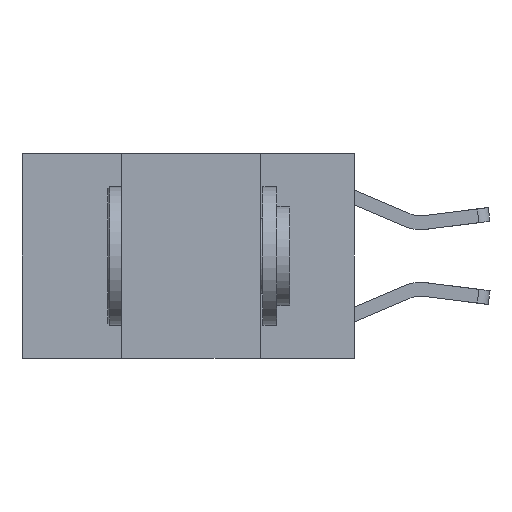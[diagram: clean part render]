
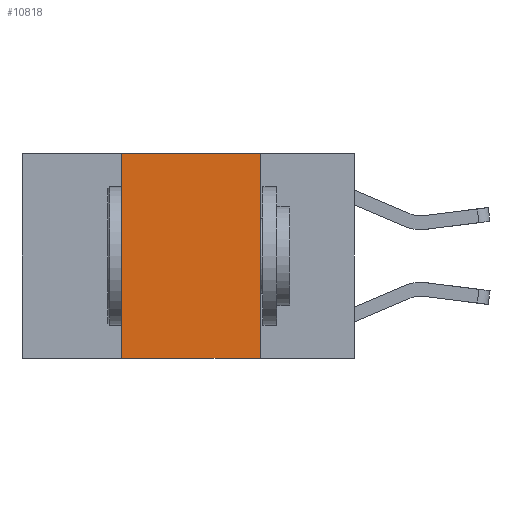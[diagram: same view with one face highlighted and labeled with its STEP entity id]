
A CAD part, left-side view. The second image highlights one B-rep face of the part: STEP entity #10818.
In plain terms, the highlighted planar face has unit normal (-1, 0, 0).
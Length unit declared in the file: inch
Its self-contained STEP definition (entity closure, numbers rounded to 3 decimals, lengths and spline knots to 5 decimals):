
#164 = PLANE ( 'NONE',  #9741 ) ;
#352 = LINE ( 'NONE', #2138, #2866 ) ;
#410 = ORIENTED_EDGE ( 'NONE', *, *, #660, .T. ) ;
#660 = EDGE_CURVE ( 'NONE', #4712, #5488, #6547, .T. ) ;
#1065 = EDGE_LOOP ( 'NONE', ( #1125, #4138, #1600, #410 ) ) ;
#1125 = ORIENTED_EDGE ( 'NONE', *, *, #5819, .F. ) ;
#1174 = DIRECTION ( 'NONE',  ( 0., 0., -1. ) ) ;
#1600 = ORIENTED_EDGE ( 'NONE', *, *, #7904, .F. ) ;
#2138 = CARTESIAN_POINT ( 'NONE',  ( 0., 0.6, 0. ) ) ;
#2260 = CARTESIAN_POINT ( 'NONE',  ( 0., 0.17, 0. ) ) ;
#2429 = DIRECTION ( 'NONE',  ( 0., -1., 0. ) ) ;
#2845 = EDGE_CURVE ( 'NONE', #5716, #3386, #352, .T. ) ;
#2866 = VECTOR ( 'NONE', #2429, 39.37008 ) ;
#3131 = DIRECTION ( 'NONE',  ( 0., 0., -1. ) ) ;
#3260 = CARTESIAN_POINT ( 'NONE',  ( 0., 0.17, 0. ) ) ;
#3386 = VERTEX_POINT ( 'NONE', #3260 ) ;
#3578 = DIRECTION ( 'NONE',  ( 0., 0., 1. ) ) ;
#4138 = ORIENTED_EDGE ( 'NONE', *, *, #2845, .F. ) ;
#4712 = VERTEX_POINT ( 'NONE', #9604 ) ;
#4734 = LINE ( 'NONE', #8833, #7087 ) ;
#5488 = VERTEX_POINT ( 'NONE', #9739 ) ;
#5716 = VERTEX_POINT ( 'NONE', #7437 ) ;
#5819 = EDGE_CURVE ( 'NONE', #3386, #5488, #9512, .T. ) ;
#6547 = LINE ( 'NONE', #10647, #8536 ) ;
#6597 = DIRECTION ( 'NONE',  ( 1., 0., 0. ) ) ;
#6972 = DIRECTION ( 'NONE',  ( 0., -1., 0. ) ) ;
#7087 = VECTOR ( 'NONE', #3578, 39.37008 ) ;
#7437 = CARTESIAN_POINT ( 'NONE',  ( 0., 0.42, 0. ) ) ;
#7904 = EDGE_CURVE ( 'NONE', #4712, #5716, #4734, .T. ) ;
#7917 = FACE_OUTER_BOUND ( 'NONE', #1065, .T. ) ;
#8536 = VECTOR ( 'NONE', #6972, 39.37008 ) ;
#8833 = CARTESIAN_POINT ( 'NONE',  ( 0., 0.42, 0. ) ) ;
#9512 = LINE ( 'NONE', #2260, #11208 ) ;
#9604 = CARTESIAN_POINT ( 'NONE',  ( 0., 0.42, -0.37 ) ) ;
#9739 = CARTESIAN_POINT ( 'NONE',  ( 0., 0.17, -0.37 ) ) ;
#9741 = AXIS2_PLACEMENT_3D ( 'NONE', #10815, #6597, #1174 ) ;
#10647 = CARTESIAN_POINT ( 'NONE',  ( 0., 0.6, -0.37 ) ) ;
#10815 = CARTESIAN_POINT ( 'NONE',  ( 0., 0.6, 0. ) ) ;
#10818 = ADVANCED_FACE ( 'NONE', ( #7917 ), #164, .F. ) ;
#11208 = VECTOR ( 'NONE', #3131, 39.37008 ) ;
